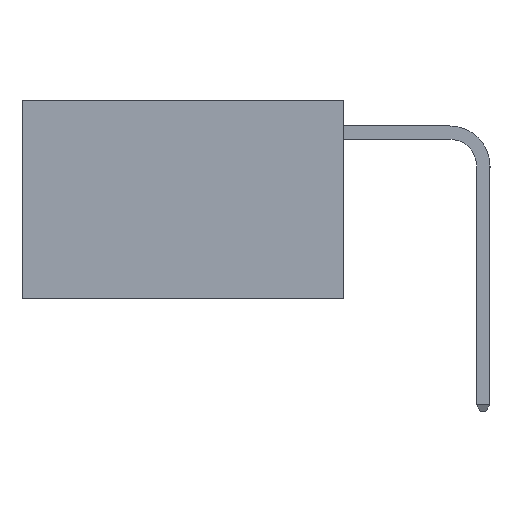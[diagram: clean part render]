
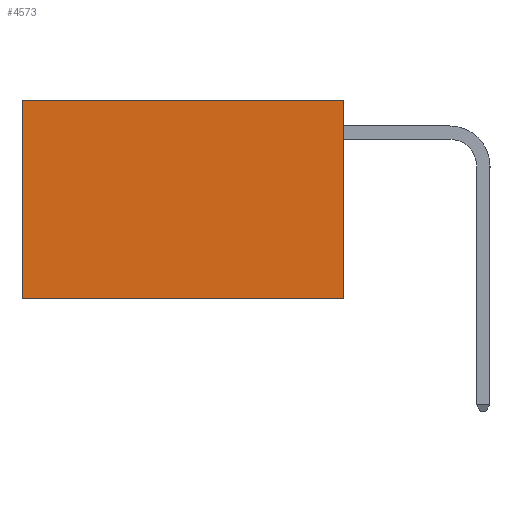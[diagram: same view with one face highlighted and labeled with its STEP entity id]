
A CAD part, left-side view. The second image highlights one B-rep face of the part: STEP entity #4573.
In plain terms, the highlighted planar face has unit normal (-1, 0, 0).
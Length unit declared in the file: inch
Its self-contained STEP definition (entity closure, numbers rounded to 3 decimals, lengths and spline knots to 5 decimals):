
#40 = VERTEX_POINT ( 'NONE', #2939 ) ;
#133 = VECTOR ( 'NONE', #6456, 39.37008 ) ;
#135 = VERTEX_POINT ( 'NONE', #283 ) ;
#283 = CARTESIAN_POINT ( 'NONE',  ( 0.2625, 0.6, 0. ) ) ;
#825 = FACE_OUTER_BOUND ( 'NONE', #841, .T. ) ;
#841 = EDGE_LOOP ( 'NONE', ( #5996, #8808, #3553, #11821 ) ) ;
#906 = VERTEX_POINT ( 'NONE', #10589 ) ;
#1942 = DIRECTION ( 'NONE',  ( 0., 1., 0. ) ) ;
#2031 = CARTESIAN_POINT ( 'NONE',  ( 0.2625, 0.6, 0. ) ) ;
#2733 = VECTOR ( 'NONE', #9413, 39.37008 ) ;
#2939 = CARTESIAN_POINT ( 'NONE',  ( 0.2625, 0., -0.37 ) ) ;
#3017 = LINE ( 'NONE', #10592, #133 ) ;
#3075 = AXIS2_PLACEMENT_3D ( 'NONE', #7847, #5786, #12970 ) ;
#3553 = ORIENTED_EDGE ( 'NONE', *, *, #9642, .F. ) ;
#3819 = VERTEX_POINT ( 'NONE', #5389 ) ;
#3953 = LINE ( 'NONE', #7634, #11894 ) ;
#4573 = ADVANCED_FACE ( 'NONE', ( #825 ), #4718, .F. ) ;
#4718 = PLANE ( 'NONE',  #3075 ) ;
#4809 = VECTOR ( 'NONE', #1942, 39.37008 ) ;
#5389 = CARTESIAN_POINT ( 'NONE',  ( 0.2625, 0., 0. ) ) ;
#5420 = EDGE_CURVE ( 'NONE', #3819, #135, #7940, .T. ) ;
#5786 = DIRECTION ( 'NONE',  ( 1., 0., 0. ) ) ;
#5996 = ORIENTED_EDGE ( 'NONE', *, *, #8074, .T. ) ;
#6456 = DIRECTION ( 'NONE',  ( 0., 1., 0. ) ) ;
#7634 = CARTESIAN_POINT ( 'NONE',  ( 0.2625, 0., 0. ) ) ;
#7847 = CARTESIAN_POINT ( 'NONE',  ( 0.2625, 0., 0. ) ) ;
#7940 = LINE ( 'NONE', #12313, #4809 ) ;
#8074 = EDGE_CURVE ( 'NONE', #135, #906, #13440, .T. ) ;
#8707 = DIRECTION ( 'NONE',  ( 0., 0., -1. ) ) ;
#8808 = ORIENTED_EDGE ( 'NONE', *, *, #13071, .F. ) ;
#9413 = DIRECTION ( 'NONE',  ( 0., 0., -1. ) ) ;
#9642 = EDGE_CURVE ( 'NONE', #3819, #40, #3953, .T. ) ;
#10589 = CARTESIAN_POINT ( 'NONE',  ( 0.2625, 0.6, -0.37 ) ) ;
#10592 = CARTESIAN_POINT ( 'NONE',  ( 0.2625, 0., -0.37 ) ) ;
#11821 = ORIENTED_EDGE ( 'NONE', *, *, #5420, .T. ) ;
#11894 = VECTOR ( 'NONE', #8707, 39.37008 ) ;
#12313 = CARTESIAN_POINT ( 'NONE',  ( 0.2625, 0., 0. ) ) ;
#12970 = DIRECTION ( 'NONE',  ( 0., 0., -1. ) ) ;
#13071 = EDGE_CURVE ( 'NONE', #40, #906, #3017, .T. ) ;
#13440 = LINE ( 'NONE', #2031, #2733 ) ;
